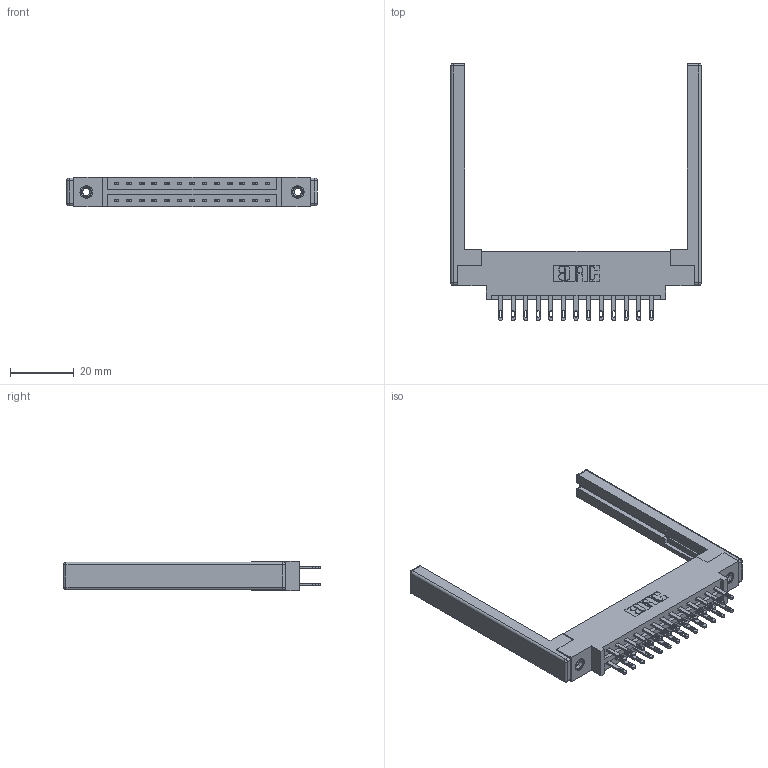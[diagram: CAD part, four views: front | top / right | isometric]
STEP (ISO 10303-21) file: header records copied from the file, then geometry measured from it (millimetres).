
FILE_DESCRIPTION (( 'STEP AP203' ), '1' );
FILE_NAME ('337-026-500-868.STEP', '2019-10-10T21:28:41', ( '' ), ( '' ), 'SwSTEP 2.0', 'SolidWorks 2016', '' );
FILE_SCHEMA (( 'CONFIG_CONTROL_DESIGN' ));
Length unit declared in the file: inch
Products named in the file (5): 337 Part_0.170 Offset - 0.156 Dia-TI; 337-026-500-868; 307-220-068; 345-292-001_345-293-100; 345-250-001_345-250-001-102
Assembly tree (31 placements, depth 2):
  337-026-500-868
    337 Part_0.170 Offset - 0.156 Dia-TI
    345-292-001_345-293-100  x26
    345-250-001_345-250-001-102  x2
    307-220-068  x2
Bounding box: 78.94 x 80.9 x 9.4 mm (x, y, z)
Volume: 12280.4 mm3; surface area: 13075 mm2
Topology: 31 solids, 31 shells, 1572 faces, 4691 edges, 3106 vertices
Faces by surface type: plane 994, cylinder 554, cone 12, sphere 8, torus 4
Entity records: 16652 total; most frequent: CARTESIAN_POINT 2795, ORIENTED_EDGE 2720, DIRECTION 2502, EDGE_CURVE 1360, VECTOR 1178, LINE 1178, VERTEX_POINT 898, AXIS2_PLACEMENT_3D 662
